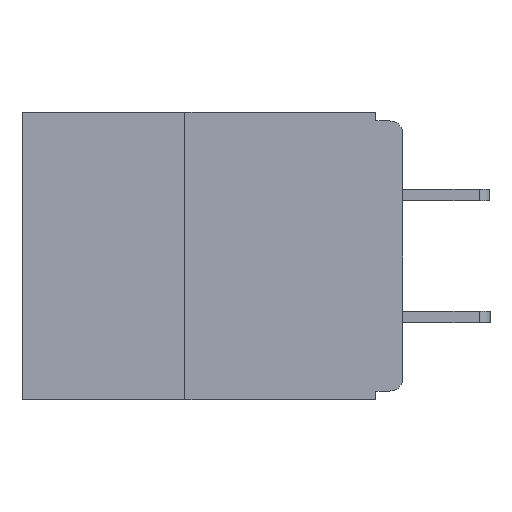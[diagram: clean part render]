
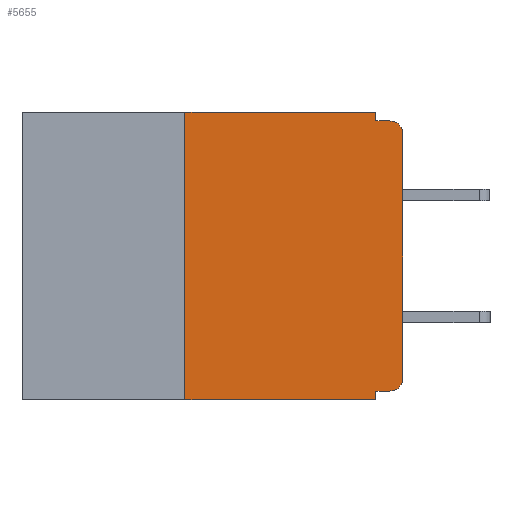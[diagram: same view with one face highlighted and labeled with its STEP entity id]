
A CAD part, left-side view. The second image highlights one B-rep face of the part: STEP entity #5655.
In plain terms, the highlighted planar face has unit normal (-1, 0, 0).
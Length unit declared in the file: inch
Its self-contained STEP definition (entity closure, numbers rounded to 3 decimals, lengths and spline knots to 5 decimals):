
#138 = EDGE_CURVE ( 'NONE', #9997, #1355, #11465, .T. ) ;
#170 = CARTESIAN_POINT ( 'NONE',  ( 0., 0., -0.01 ) ) ;
#203 = CARTESIAN_POINT ( 'NONE',  ( 0., 0.031, -0.33 ) ) ;
#215 = EDGE_LOOP ( 'NONE', ( #6634, #3488, #3288, #3019, #1425, #599, #5070, #11674, #7106, #6673 ) ) ;
#236 = DIRECTION ( 'NONE',  ( 0., -1., 0. ) ) ;
#392 = EDGE_CURVE ( 'NONE', #4465, #2598, #1496, .T. ) ;
#599 = ORIENTED_EDGE ( 'NONE', *, *, #4120, .F. ) ;
#832 = CIRCLE ( 'NONE', #5824, 0.015 ) ;
#912 = EDGE_CURVE ( 'NONE', #2448, #8759, #7215, .T. ) ;
#915 = CARTESIAN_POINT ( 'NONE',  ( 0., 0.031, -0.33 ) ) ;
#1243 = EDGE_CURVE ( 'NONE', #1355, #2598, #832, .T. ) ;
#1355 = VERTEX_POINT ( 'NONE', #10552 ) ;
#1357 = VECTOR ( 'NONE', #4031, 39.37008 ) ;
#1383 = LINE ( 'NONE', #2824, #11282 ) ;
#1425 = ORIENTED_EDGE ( 'NONE', *, *, #10708, .F. ) ;
#1496 = LINE ( 'NONE', #170, #4426 ) ;
#1617 = CARTESIAN_POINT ( 'NONE',  ( 0., 0.437, 0. ) ) ;
#1916 = VECTOR ( 'NONE', #10454, 39.37008 ) ;
#1924 = EDGE_CURVE ( 'NONE', #2448, #9997, #11214, .T. ) ;
#2076 = CARTESIAN_POINT ( 'NONE',  ( 0., 0.25, -0.33 ) ) ;
#2179 = LINE ( 'NONE', #7069, #5355 ) ;
#2448 = VERTEX_POINT ( 'NONE', #8757 ) ;
#2513 = AXIS2_PLACEMENT_3D ( 'NONE', #4649, #4629, #7509 ) ;
#2548 = CARTESIAN_POINT ( 'NONE',  ( 0., 0.25, 0. ) ) ;
#2598 = VERTEX_POINT ( 'NONE', #12040 ) ;
#2824 = CARTESIAN_POINT ( 'NONE',  ( 0., 0.437, -0.33 ) ) ;
#3019 = ORIENTED_EDGE ( 'NONE', *, *, #3961, .F. ) ;
#3096 = VECTOR ( 'NONE', #5805, 39.37008 ) ;
#3288 = ORIENTED_EDGE ( 'NONE', *, *, #392, .F. ) ;
#3488 = ORIENTED_EDGE ( 'NONE', *, *, #1243, .T. ) ;
#3601 = DIRECTION ( 'NONE',  ( 1., 0., 0. ) ) ;
#3961 = EDGE_CURVE ( 'NONE', #7059, #4465, #9218, .T. ) ;
#4031 = DIRECTION ( 'NONE',  ( 0., -1., 0. ) ) ;
#4120 = EDGE_CURVE ( 'NONE', #9346, #4891, #2179, .T. ) ;
#4426 = VECTOR ( 'NONE', #236, 39.37008 ) ;
#4446 = EDGE_CURVE ( 'NONE', #9346, #7427, #1383, .T. ) ;
#4465 = VERTEX_POINT ( 'NONE', #4777 ) ;
#4528 = EDGE_CURVE ( 'NONE', #8759, #7427, #5945, .T. ) ;
#4629 = DIRECTION ( 'NONE',  ( -1., 0., 0. ) ) ;
#4649 = CARTESIAN_POINT ( 'NONE',  ( 0., 0.015, -0.305 ) ) ;
#4777 = CARTESIAN_POINT ( 'NONE',  ( 0., 0.031, -0.01 ) ) ;
#4891 = VERTEX_POINT ( 'NONE', #2548 ) ;
#5070 = ORIENTED_EDGE ( 'NONE', *, *, #4446, .T. ) ;
#5183 = DIRECTION ( 'NONE',  ( 0., 0., -1. ) ) ;
#5355 = VECTOR ( 'NONE', #8880, 39.37008 ) ;
#5617 = CARTESIAN_POINT ( 'NONE',  ( 0., 0.015, -0.025 ) ) ;
#5655 = ADVANCED_FACE ( 'NONE', ( #10840 ), #9155, .F. ) ;
#5805 = DIRECTION ( 'NONE',  ( 0., 0., -1. ) ) ;
#5824 = AXIS2_PLACEMENT_3D ( 'NONE', #5617, #12052, #5183 ) ;
#5945 = LINE ( 'NONE', #915, #3096 ) ;
#6634 = ORIENTED_EDGE ( 'NONE', *, *, #138, .T. ) ;
#6658 = DIRECTION ( 'NONE',  ( 0., 1., 0. ) ) ;
#6673 = ORIENTED_EDGE ( 'NONE', *, *, #1924, .T. ) ;
#6685 = CARTESIAN_POINT ( 'NONE',  ( 0., 0., 0. ) ) ;
#6849 = DIRECTION ( 'NONE',  ( 0., 0., -1. ) ) ;
#7059 = VERTEX_POINT ( 'NONE', #11066 ) ;
#7069 = CARTESIAN_POINT ( 'NONE',  ( 0., 0.25, -0.33 ) ) ;
#7106 = ORIENTED_EDGE ( 'NONE', *, *, #912, .F. ) ;
#7215 = LINE ( 'NONE', #11921, #11105 ) ;
#7427 = VERTEX_POINT ( 'NONE', #203 ) ;
#7509 = DIRECTION ( 'NONE',  ( 0., 0., -1. ) ) ;
#7741 = CARTESIAN_POINT ( 'NONE',  ( 0., 0.031, 0. ) ) ;
#7883 = CARTESIAN_POINT ( 'NONE',  ( 0., 0.031, -0.32 ) ) ;
#8757 = CARTESIAN_POINT ( 'NONE',  ( 0., 0.015, -0.32 ) ) ;
#8759 = VERTEX_POINT ( 'NONE', #7883 ) ;
#8880 = DIRECTION ( 'NONE',  ( 0., 0., 1. ) ) ;
#8945 = VECTOR ( 'NONE', #6849, 39.37008 ) ;
#9155 = PLANE ( 'NONE',  #10690 ) ;
#9218 = LINE ( 'NONE', #7741, #8945 ) ;
#9333 = DIRECTION ( 'NONE',  ( 0., -1., 0. ) ) ;
#9346 = VERTEX_POINT ( 'NONE', #2076 ) ;
#9997 = VERTEX_POINT ( 'NONE', #11284 ) ;
#10022 = DIRECTION ( 'NONE',  ( 0., 0., -1. ) ) ;
#10407 = CARTESIAN_POINT ( 'NONE',  ( 0., 0.437, 0. ) ) ;
#10454 = DIRECTION ( 'NONE',  ( 0., 0., 1. ) ) ;
#10552 = CARTESIAN_POINT ( 'NONE',  ( 0., 0., -0.025 ) ) ;
#10690 = AXIS2_PLACEMENT_3D ( 'NONE', #1617, #3601, #10022 ) ;
#10708 = EDGE_CURVE ( 'NONE', #4891, #7059, #11260, .T. ) ;
#10840 = FACE_OUTER_BOUND ( 'NONE', #215, .T. ) ;
#11066 = CARTESIAN_POINT ( 'NONE',  ( 0., 0.031, 0. ) ) ;
#11105 = VECTOR ( 'NONE', #6658, 39.37008 ) ;
#11214 = CIRCLE ( 'NONE', #2513, 0.015 ) ;
#11260 = LINE ( 'NONE', #10407, #1357 ) ;
#11282 = VECTOR ( 'NONE', #9333, 39.37008 ) ;
#11284 = CARTESIAN_POINT ( 'NONE',  ( 0., 0., -0.305 ) ) ;
#11465 = LINE ( 'NONE', #6685, #1916 ) ;
#11674 = ORIENTED_EDGE ( 'NONE', *, *, #4528, .F. ) ;
#11921 = CARTESIAN_POINT ( 'NONE',  ( 0., 0., -0.32 ) ) ;
#12040 = CARTESIAN_POINT ( 'NONE',  ( 0., 0.015, -0.01 ) ) ;
#12052 = DIRECTION ( 'NONE',  ( -1., 0., 0. ) ) ;
